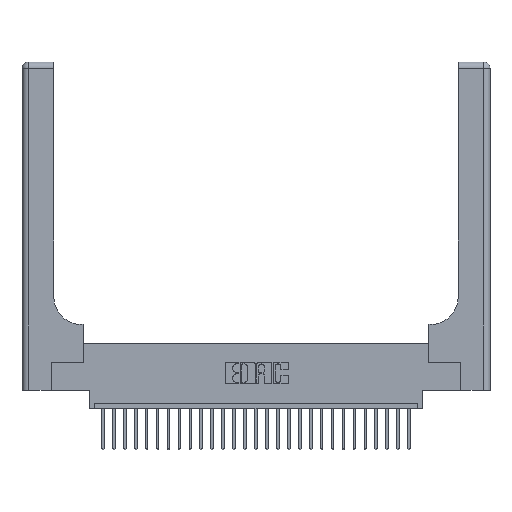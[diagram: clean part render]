
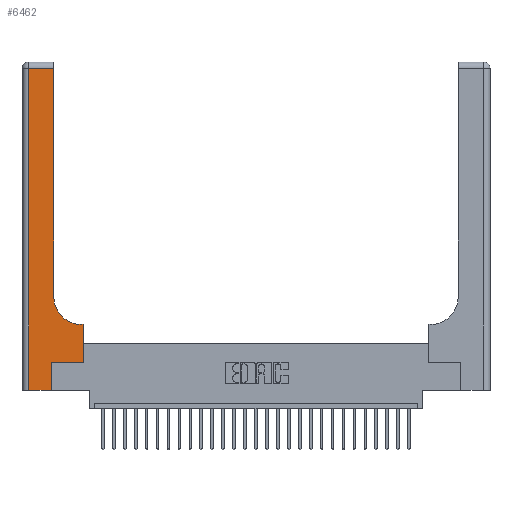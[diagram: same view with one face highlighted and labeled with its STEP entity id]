
A CAD part, top view. The second image highlights one B-rep face of the part: STEP entity #6462.
In plain terms, the highlighted planar face has unit normal (0, 0, 1).
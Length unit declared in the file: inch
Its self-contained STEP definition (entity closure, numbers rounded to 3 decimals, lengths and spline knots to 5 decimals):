
#17 = CARTESIAN_POINT ( 'NONE',  ( 0., 2.94, 0.37 ) ) ;
#215 = CARTESIAN_POINT ( 'NONE',  ( 0.5585, 0.25, 0.37 ) ) ;
#269 = ORIENTED_EDGE ( 'NONE', *, *, #5714, .T. ) ;
#277 = AXIS2_PLACEMENT_3D ( 'NONE', #17506, #15330, #22329 ) ;
#767 = CARTESIAN_POINT ( 'NONE',  ( 0.269, 0.25, 0.37 ) ) ;
#1057 = VECTOR ( 'NONE', #4905, 39.37008 ) ;
#1565 = EDGE_CURVE ( 'NONE', #12633, #21951, #27239, .T. ) ;
#2111 = DIRECTION ( 'NONE',  ( -1., 0., 0. ) ) ;
#3391 = VECTOR ( 'NONE', #5012, 39.37008 ) ;
#3429 = LINE ( 'NONE', #12179, #18413 ) ;
#3521 = DIRECTION ( 'NONE',  ( 0., -1., 0. ) ) ;
#3538 = VECTOR ( 'NONE', #21652, 39.37008 ) ;
#4102 = LINE ( 'NONE', #767, #3391 ) ;
#4243 = DIRECTION ( 'NONE',  ( 0., 1., 0. ) ) ;
#4401 = CARTESIAN_POINT ( 'NONE',  ( 0.5585, 0.6, 0.37 ) ) ;
#4905 = DIRECTION ( 'NONE',  ( -1., 0., 0. ) ) ;
#4963 = CARTESIAN_POINT ( 'NONE',  ( 0.5585, 0.25, 0.37 ) ) ;
#5012 = DIRECTION ( 'NONE',  ( 1., 0., 0. ) ) ;
#5533 = ORIENTED_EDGE ( 'NONE', *, *, #24979, .T. ) ;
#5601 = LINE ( 'NONE', #6465, #9785 ) ;
#5714 = EDGE_CURVE ( 'NONE', #15353, #28280, #19313, .T. ) ;
#5789 = VERTEX_POINT ( 'NONE', #26185 ) ;
#6401 = EDGE_CURVE ( 'NONE', #14948, #5789, #14300, .T. ) ;
#6448 = DIRECTION ( 'NONE',  ( 0., 0., -1. ) ) ;
#6462 = ADVANCED_FACE ( 'NONE', ( #18522 ), #19853, .F. ) ;
#6465 = CARTESIAN_POINT ( 'NONE',  ( 0.2915, 3., 0.37 ) ) ;
#6664 = CARTESIAN_POINT ( 'NONE',  ( 0.2915, 0.6, 0.37 ) ) ;
#6693 = VERTEX_POINT ( 'NONE', #19746 ) ;
#6839 = EDGE_CURVE ( 'NONE', #21951, #14948, #23799, .T. ) ;
#7313 = VERTEX_POINT ( 'NONE', #12622 ) ;
#7410 = VECTOR ( 'NONE', #20597, 39.37008 ) ;
#7760 = ORIENTED_EDGE ( 'NONE', *, *, #12440, .T. ) ;
#8833 = CARTESIAN_POINT ( 'NONE',  ( 0., 0., 0.37 ) ) ;
#9785 = VECTOR ( 'NONE', #4243, 39.37008 ) ;
#11054 = CARTESIAN_POINT ( 'NONE',  ( 0.269, 0.25, 0.37 ) ) ;
#11251 = CARTESIAN_POINT ( 'NONE',  ( 0.06, 0., 0.37 ) ) ;
#11751 = VECTOR ( 'NONE', #27383, 39.37008 ) ;
#12179 = CARTESIAN_POINT ( 'NONE',  ( 0.269, 0., 0.37 ) ) ;
#12440 = EDGE_CURVE ( 'NONE', #20994, #15353, #4102, .T. ) ;
#12622 = CARTESIAN_POINT ( 'NONE',  ( 0.2915, 0.85, 0.37 ) ) ;
#12633 = VERTEX_POINT ( 'NONE', #21351 ) ;
#13819 = ORIENTED_EDGE ( 'NONE', *, *, #18736, .T. ) ;
#14300 = LINE ( 'NONE', #8833, #3538 ) ;
#14948 = VERTEX_POINT ( 'NONE', #11251 ) ;
#15330 = DIRECTION ( 'NONE',  ( 0., 0., -1. ) ) ;
#15353 = VERTEX_POINT ( 'NONE', #215 ) ;
#15424 = CARTESIAN_POINT ( 'NONE',  ( 0., 3., 0.37 ) ) ;
#15729 = EDGE_CURVE ( 'NONE', #28280, #6693, #25412, .T. ) ;
#15802 = ORIENTED_EDGE ( 'NONE', *, *, #6401, .T. ) ;
#15804 = EDGE_CURVE ( 'NONE', #5789, #20994, #3429, .T. ) ;
#17506 = CARTESIAN_POINT ( 'NONE',  ( 0.5415, 0.85, 0.37 ) ) ;
#18413 = VECTOR ( 'NONE', #20922, 39.37008 ) ;
#18522 = FACE_OUTER_BOUND ( 'NONE', #18649, .T. ) ;
#18649 = EDGE_LOOP ( 'NONE', ( #5533, #23157, #19119, #15802, #26155, #7760, #269, #28572, #13819 ) ) ;
#18736 = EDGE_CURVE ( 'NONE', #6693, #7313, #26011, .T. ) ;
#19119 = ORIENTED_EDGE ( 'NONE', *, *, #6839, .T. ) ;
#19313 = LINE ( 'NONE', #4963, #7410 ) ;
#19746 = CARTESIAN_POINT ( 'NONE',  ( 0.5415, 0.6, 0.37 ) ) ;
#19853 = PLANE ( 'NONE',  #25882 ) ;
#20597 = DIRECTION ( 'NONE',  ( 0., 1., 0. ) ) ;
#20922 = DIRECTION ( 'NONE',  ( 0., 1., 0. ) ) ;
#20994 = VERTEX_POINT ( 'NONE', #11054 ) ;
#21351 = CARTESIAN_POINT ( 'NONE',  ( 0.2915, 2.94, 0.37 ) ) ;
#21652 = DIRECTION ( 'NONE',  ( 1., 0., 0. ) ) ;
#21951 = VERTEX_POINT ( 'NONE', #23909 ) ;
#22329 = DIRECTION ( 'NONE',  ( 1., 0., 0. ) ) ;
#23157 = ORIENTED_EDGE ( 'NONE', *, *, #1565, .T. ) ;
#23460 = VECTOR ( 'NONE', #3521, 39.37008 ) ;
#23799 = LINE ( 'NONE', #27945, #23460 ) ;
#23909 = CARTESIAN_POINT ( 'NONE',  ( 0.06, 2.94, 0.37 ) ) ;
#24979 = EDGE_CURVE ( 'NONE', #7313, #12633, #5601, .T. ) ;
#25412 = LINE ( 'NONE', #6664, #11751 ) ;
#25882 = AXIS2_PLACEMENT_3D ( 'NONE', #15424, #6448, #2111 ) ;
#26011 = CIRCLE ( 'NONE', #277, 0.25 ) ;
#26155 = ORIENTED_EDGE ( 'NONE', *, *, #15804, .T. ) ;
#26185 = CARTESIAN_POINT ( 'NONE',  ( 0.269, 0., 0.37 ) ) ;
#27239 = LINE ( 'NONE', #17, #1057 ) ;
#27383 = DIRECTION ( 'NONE',  ( -1., 0., 0. ) ) ;
#27945 = CARTESIAN_POINT ( 'NONE',  ( 0.06, 3., 0.37 ) ) ;
#28280 = VERTEX_POINT ( 'NONE', #4401 ) ;
#28572 = ORIENTED_EDGE ( 'NONE', *, *, #15729, .T. ) ;
